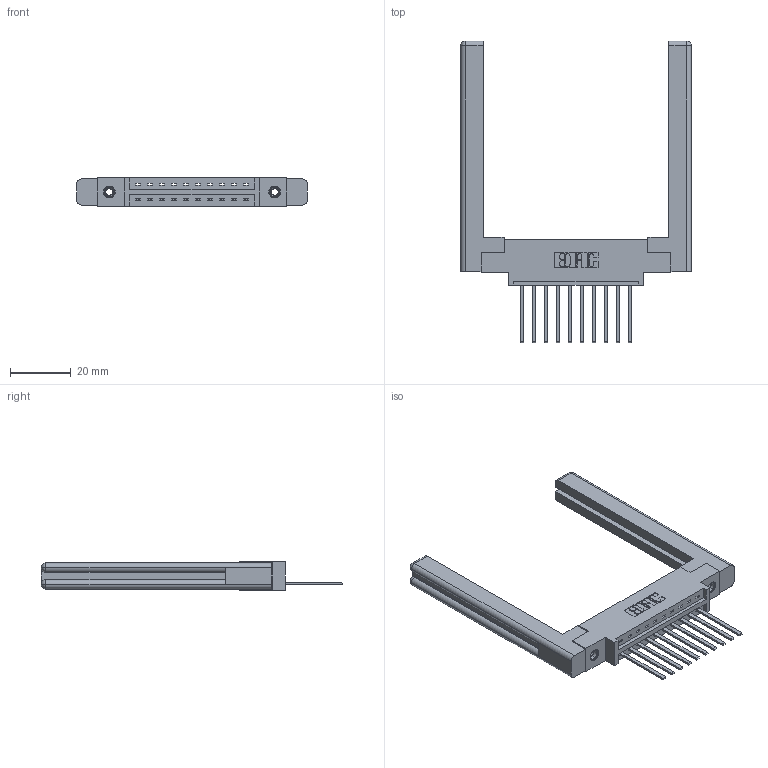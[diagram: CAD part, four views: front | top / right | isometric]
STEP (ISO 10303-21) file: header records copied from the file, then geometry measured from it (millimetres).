
FILE_DESCRIPTION (( 'STEP AP203' ), '1' );
FILE_NAME ('387-010-544-658.STEP', '2019-10-02T11:42:49', ( '' ), ( '' ), 'SwSTEP 2.0', 'SolidWorks 2016', '' );
FILE_SCHEMA (( 'CONFIG_CONTROL_DESIGN' ));
Length unit declared in the file: inch
Products named in the file (5): 387-010-544-658; 345-292-001_345-293-144; 307-220-058; 337 Part_0.170 Offset - 0.156 Dia-TI; 345-250-001_345-250-001-102
Assembly tree (15 placements, depth 2):
  387-010-544-658
    337 Part_0.170 Offset - 0.156 Dia-TI
    345-292-001_345-293-144  x10
    345-250-001_345-250-001-102  x2
    307-220-058  x2
Bounding box: 76.25 x 99.7 x 9.4 mm (x, y, z)
Volume: 14685 mm3; surface area: 13286.6 mm2
Topology: 15 solids, 15 shells, 820 faces, 2377 edges, 1558 vertices
Faces by surface type: plane 578, cylinder 218, cone 12, torus 12
Entity records: 14154 total; most frequent: CARTESIAN_POINT 2463, ORIENTED_EDGE 2348, DIRECTION 2154, EDGE_CURVE 1174, VECTOR 1002, LINE 1002, VERTEX_POINT 774, AXIS2_PLACEMENT_3D 576
